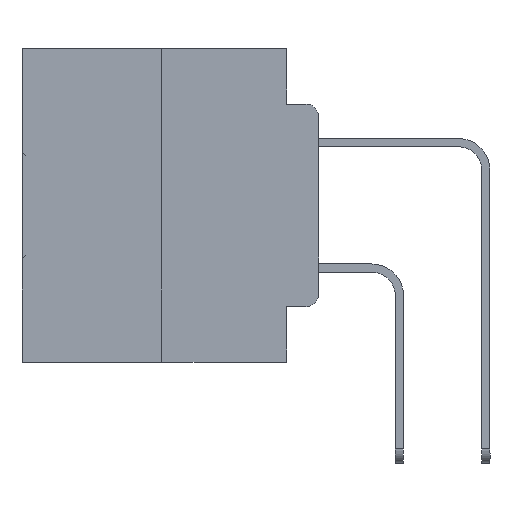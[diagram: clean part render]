
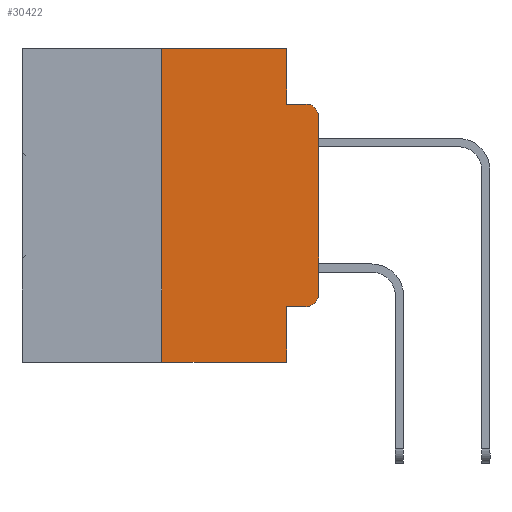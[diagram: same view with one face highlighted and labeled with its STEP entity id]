
A CAD part, left-side view. The second image highlights one B-rep face of the part: STEP entity #30422.
In plain terms, the highlighted planar face has unit normal (-1, 0, 0).
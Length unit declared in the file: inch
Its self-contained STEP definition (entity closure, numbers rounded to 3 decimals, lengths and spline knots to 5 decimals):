
#160 = VERTEX_POINT ( 'NONE', #6407 ) ;
#512 = VERTEX_POINT ( 'NONE', #11275 ) ;
#917 = CARTESIAN_POINT ( 'NONE',  ( 0., 0.051, -0.4115 ) ) ;
#1955 = AXIS2_PLACEMENT_3D ( 'NONE', #13356, #26862, #11428 ) ;
#2045 = ORIENTED_EDGE ( 'NONE', *, *, #25439, .F. ) ;
#2211 = LINE ( 'NONE', #29198, #20323 ) ;
#2756 = DIRECTION ( 'NONE',  ( 0., 0., -1. ) ) ;
#3462 = VERTEX_POINT ( 'NONE', #12000 ) ;
#3608 = DIRECTION ( 'NONE',  ( 0., 0., -1. ) ) ;
#5111 = CARTESIAN_POINT ( 'NONE',  ( 0., 0.051, -0.0885 ) ) ;
#6219 = VECTOR ( 'NONE', #27608, 39.37008 ) ;
#6251 = VECTOR ( 'NONE', #9714, 39.37008 ) ;
#6407 = CARTESIAN_POINT ( 'NONE',  ( 0., 0.25, -0.5 ) ) ;
#7383 = VECTOR ( 'NONE', #25145, 39.37008 ) ;
#8535 = EDGE_CURVE ( 'NONE', #12512, #22873, #29136, .T. ) ;
#8621 = PLANE ( 'NONE',  #1955 ) ;
#8847 = CARTESIAN_POINT ( 'NONE',  ( 0., 0.051, -0.4115 ) ) ;
#9520 = EDGE_CURVE ( 'NONE', #160, #3462, #31168, .T. ) ;
#9714 = DIRECTION ( 'NONE',  ( 0., 0., 1. ) ) ;
#10686 = VERTEX_POINT ( 'NONE', #18629 ) ;
#10707 = ORIENTED_EDGE ( 'NONE', *, *, #14210, .F. ) ;
#11086 = ORIENTED_EDGE ( 'NONE', *, *, #26651, .T. ) ;
#11275 = CARTESIAN_POINT ( 'NONE',  ( 0., 0.02, -0.4115 ) ) ;
#11428 = DIRECTION ( 'NONE',  ( 0., 0., -1. ) ) ;
#12000 = CARTESIAN_POINT ( 'NONE',  ( 0., 0.051, -0.5 ) ) ;
#12281 = ORIENTED_EDGE ( 'NONE', *, *, #21719, .T. ) ;
#12512 = VERTEX_POINT ( 'NONE', #26831 ) ;
#12669 = DIRECTION ( 'NONE',  ( 0., 0., -1. ) ) ;
#13276 = EDGE_LOOP ( 'NONE', ( #20686, #19791, #15261, #10707, #2045, #24934, #26416, #33084, #11086, #12281 ) ) ;
#13356 = CARTESIAN_POINT ( 'NONE',  ( 0., 0.473, 0. ) ) ;
#14111 = LINE ( 'NONE', #27265, #24235 ) ;
#14210 = EDGE_CURVE ( 'NONE', #28823, #12512, #14111, .T. ) ;
#14442 = CARTESIAN_POINT ( 'NONE',  ( 0., 0.473, 0. ) ) ;
#15043 = CIRCLE ( 'NONE', #31795, 0.02 ) ;
#15261 = ORIENTED_EDGE ( 'NONE', *, *, #8535, .F. ) ;
#16241 = DIRECTION ( 'NONE',  ( -1., 0., 0. ) ) ;
#17595 = CARTESIAN_POINT ( 'NONE',  ( 0., 0.051, 0. ) ) ;
#18563 = VECTOR ( 'NONE', #20588, 39.37008 ) ;
#18598 = DIRECTION ( 'NONE',  ( 0., -1., 0. ) ) ;
#18629 = CARTESIAN_POINT ( 'NONE',  ( 0., 0., -0.3915 ) ) ;
#19360 = LINE ( 'NONE', #8847, #6219 ) ;
#19534 = LINE ( 'NONE', #14442, #7383 ) ;
#19791 = ORIENTED_EDGE ( 'NONE', *, *, #27689, .T. ) ;
#20323 = VECTOR ( 'NONE', #20447, 39.37008 ) ;
#20360 = CARTESIAN_POINT ( 'NONE',  ( 0., 0.25, 0. ) ) ;
#20398 = CARTESIAN_POINT ( 'NONE',  ( 0., 0.02, -0.1085 ) ) ;
#20414 = CARTESIAN_POINT ( 'NONE',  ( 0., 0.25, 0. ) ) ;
#20447 = DIRECTION ( 'NONE',  ( 0., 0., -1. ) ) ;
#20588 = DIRECTION ( 'NONE',  ( 0., 0., 1. ) ) ;
#20590 = VECTOR ( 'NONE', #20823, 39.37008 ) ;
#20686 = ORIENTED_EDGE ( 'NONE', *, *, #25571, .T. ) ;
#20823 = DIRECTION ( 'NONE',  ( 0., -1., 0. ) ) ;
#21351 = CARTESIAN_POINT ( 'NONE',  ( 0., 0., -0.1085 ) ) ;
#21719 = EDGE_CURVE ( 'NONE', #512, #10686, #15043, .T. ) ;
#22873 = VERTEX_POINT ( 'NONE', #25961 ) ;
#23792 = VECTOR ( 'NONE', #18598, 39.37008 ) ;
#24235 = VECTOR ( 'NONE', #3608, 39.37008 ) ;
#24744 = FACE_OUTER_BOUND ( 'NONE', #13276, .T. ) ;
#24934 = ORIENTED_EDGE ( 'NONE', *, *, #25580, .F. ) ;
#25145 = DIRECTION ( 'NONE',  ( 0., -1., 0. ) ) ;
#25439 = EDGE_CURVE ( 'NONE', #34154, #28823, #19534, .T. ) ;
#25571 = EDGE_CURVE ( 'NONE', #10686, #30002, #30944, .T. ) ;
#25580 = EDGE_CURVE ( 'NONE', #160, #34154, #28475, .T. ) ;
#25825 = DIRECTION ( 'NONE',  ( -1., 0., 0. ) ) ;
#25961 = CARTESIAN_POINT ( 'NONE',  ( 0., 0.02, -0.0885 ) ) ;
#26416 = ORIENTED_EDGE ( 'NONE', *, *, #9520, .T. ) ;
#26651 = EDGE_CURVE ( 'NONE', #30522, #512, #19360, .T. ) ;
#26831 = CARTESIAN_POINT ( 'NONE',  ( 0., 0.051, -0.0885 ) ) ;
#26862 = DIRECTION ( 'NONE',  ( 1., 0., 0. ) ) ;
#27265 = CARTESIAN_POINT ( 'NONE',  ( 0., 0.051, 0. ) ) ;
#27608 = DIRECTION ( 'NONE',  ( 0., -1., 0. ) ) ;
#27689 = EDGE_CURVE ( 'NONE', #30002, #22873, #32038, .T. ) ;
#28475 = LINE ( 'NONE', #20414, #18563 ) ;
#28504 = EDGE_CURVE ( 'NONE', #30522, #3462, #2211, .T. ) ;
#28659 = AXIS2_PLACEMENT_3D ( 'NONE', #20398, #25825, #12669 ) ;
#28823 = VERTEX_POINT ( 'NONE', #17595 ) ;
#29136 = LINE ( 'NONE', #5111, #23792 ) ;
#29198 = CARTESIAN_POINT ( 'NONE',  ( 0., 0.051, 0. ) ) ;
#29577 = CARTESIAN_POINT ( 'NONE',  ( 0., 0.02, -0.3915 ) ) ;
#30002 = VERTEX_POINT ( 'NONE', #21351 ) ;
#30422 = ADVANCED_FACE ( 'NONE', ( #24744 ), #8621, .F. ) ;
#30522 = VERTEX_POINT ( 'NONE', #917 ) ;
#30944 = LINE ( 'NONE', #34095, #6251 ) ;
#31168 = LINE ( 'NONE', #31515, #20590 ) ;
#31515 = CARTESIAN_POINT ( 'NONE',  ( 0., 0.473, -0.5 ) ) ;
#31795 = AXIS2_PLACEMENT_3D ( 'NONE', #29577, #16241, #2756 ) ;
#32038 = CIRCLE ( 'NONE', #28659, 0.02 ) ;
#33084 = ORIENTED_EDGE ( 'NONE', *, *, #28504, .F. ) ;
#34095 = CARTESIAN_POINT ( 'NONE',  ( 0., 0., 0. ) ) ;
#34154 = VERTEX_POINT ( 'NONE', #20360 ) ;
